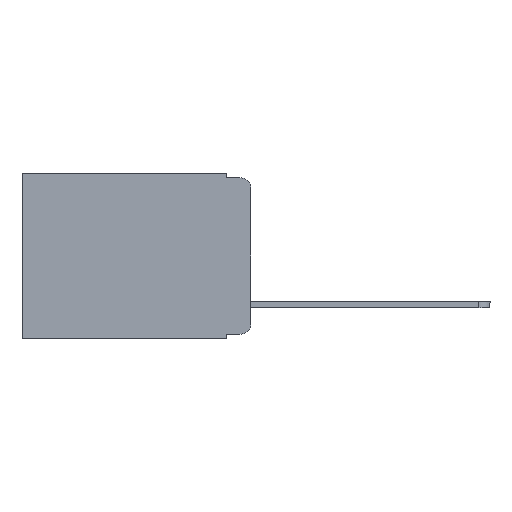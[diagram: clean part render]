
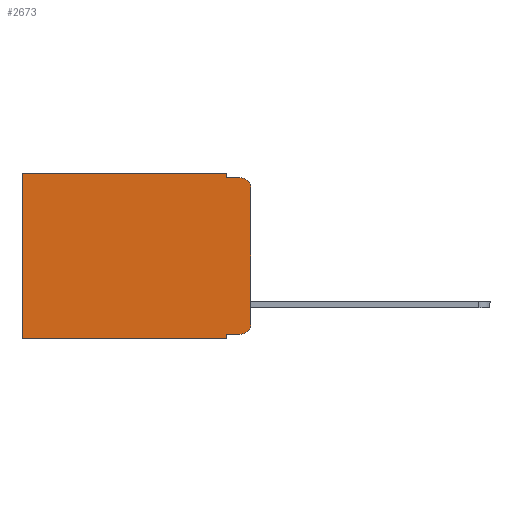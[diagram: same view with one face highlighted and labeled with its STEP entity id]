
A CAD part, left-side view. The second image highlights one B-rep face of the part: STEP entity #2673.
In plain terms, the highlighted planar face has unit normal (-1, 0, 0).
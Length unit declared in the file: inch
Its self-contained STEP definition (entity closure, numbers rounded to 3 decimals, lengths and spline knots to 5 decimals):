
#944 = VECTOR ( 'NONE', #15395, 39.37008 ) ;
#1008 = VERTEX_POINT ( 'NONE', #15096 ) ;
#1097 = DIRECTION ( 'NONE',  ( 0., 0., -1. ) ) ;
#1245 = VECTOR ( 'NONE', #19714, 39.37008 ) ;
#1649 = EDGE_CURVE ( 'NONE', #9801, #5990, #6736, .T. ) ;
#1655 = DIRECTION ( 'NONE',  ( 0., 0., -1. ) ) ;
#1959 = VERTEX_POINT ( 'NONE', #6568 ) ;
#2218 = EDGE_CURVE ( 'NONE', #9801, #3393, #4034, .T. ) ;
#2263 = CARTESIAN_POINT ( 'NONE',  ( 0.298, 0.02, -0.333 ) ) ;
#2331 = ORIENTED_EDGE ( 'NONE', *, *, #2218, .F. ) ;
#2642 = VECTOR ( 'NONE', #21369, 39.37008 ) ;
#2658 = EDGE_CURVE ( 'NONE', #5990, #1959, #10493, .T. ) ;
#2673 = ADVANCED_FACE ( 'NONE', ( #18002 ), #17777, .F. ) ;
#3393 = VERTEX_POINT ( 'NONE', #3511 ) ;
#3511 = CARTESIAN_POINT ( 'NONE',  ( 0.298, 0.051, -0.343 ) ) ;
#3837 = EDGE_LOOP ( 'NONE', ( #21745, #6970, #10984, #18626, #10590, #21558, #14095, #2331, #8886, #9224 ) ) ;
#4034 = LINE ( 'NONE', #4265, #10787 ) ;
#4265 = CARTESIAN_POINT ( 'NONE',  ( 0.298, 0.051, 0. ) ) ;
#5138 = CARTESIAN_POINT ( 'NONE',  ( 0.298, 0.051, -0.333 ) ) ;
#5890 = VECTOR ( 'NONE', #20852, 39.37008 ) ;
#5990 = VERTEX_POINT ( 'NONE', #2263 ) ;
#6135 = CARTESIAN_POINT ( 'NONE',  ( 0.298, 0.051, -0.01 ) ) ;
#6185 = DIRECTION ( 'NONE',  ( 0., 0., -1. ) ) ;
#6568 = CARTESIAN_POINT ( 'NONE',  ( 0.298, 0., -0.313 ) ) ;
#6736 = LINE ( 'NONE', #5138, #944 ) ;
#6970 = ORIENTED_EDGE ( 'NONE', *, *, #21407, .T. ) ;
#7196 = VERTEX_POINT ( 'NONE', #8000 ) ;
#7890 = CARTESIAN_POINT ( 'NONE',  ( 0.298, 0., 0. ) ) ;
#8000 = CARTESIAN_POINT ( 'NONE',  ( 0.298, 0.02, -0.01 ) ) ;
#8391 = CARTESIAN_POINT ( 'NONE',  ( 0.298, 0.051, 0. ) ) ;
#8419 = CARTESIAN_POINT ( 'NONE',  ( 0.298, 0.473, -0.343 ) ) ;
#8500 = CARTESIAN_POINT ( 'NONE',  ( 0.298, 0.473, 0. ) ) ;
#8886 = ORIENTED_EDGE ( 'NONE', *, *, #1649, .T. ) ;
#8892 = EDGE_CURVE ( 'NONE', #18422, #7196, #21714, .T. ) ;
#8947 = LINE ( 'NONE', #12167, #9162 ) ;
#9162 = VECTOR ( 'NONE', #22509, 39.37008 ) ;
#9224 = ORIENTED_EDGE ( 'NONE', *, *, #2658, .T. ) ;
#9284 = AXIS2_PLACEMENT_3D ( 'NONE', #12581, #17235, #1655 ) ;
#9745 = LINE ( 'NONE', #16690, #11934 ) ;
#9801 = VERTEX_POINT ( 'NONE', #18343 ) ;
#10105 = VECTOR ( 'NONE', #22389, 39.37008 ) ;
#10493 = CIRCLE ( 'NONE', #19944, 0.02 ) ;
#10590 = ORIENTED_EDGE ( 'NONE', *, *, #17525, .T. ) ;
#10622 = EDGE_CURVE ( 'NONE', #20757, #18422, #9745, .T. ) ;
#10787 = VECTOR ( 'NONE', #12949, 39.37008 ) ;
#10984 = ORIENTED_EDGE ( 'NONE', *, *, #8892, .F. ) ;
#11254 = VERTEX_POINT ( 'NONE', #17663 ) ;
#11306 = LINE ( 'NONE', #12683, #1245 ) ;
#11934 = VECTOR ( 'NONE', #1097, 39.37008 ) ;
#12167 = CARTESIAN_POINT ( 'NONE',  ( 0.298, 0., 0. ) ) ;
#12581 = CARTESIAN_POINT ( 'NONE',  ( 0.298, 0.02, -0.03 ) ) ;
#12683 = CARTESIAN_POINT ( 'NONE',  ( 0.298, 0., -0.343 ) ) ;
#12922 = DIRECTION ( 'NONE',  ( 1., 0., 0. ) ) ;
#12949 = DIRECTION ( 'NONE',  ( 0., 0., -1. ) ) ;
#13025 = EDGE_CURVE ( 'NONE', #11254, #22288, #19289, .T. ) ;
#13443 = AXIS2_PLACEMENT_3D ( 'NONE', #7890, #12922, #6185 ) ;
#14095 = ORIENTED_EDGE ( 'NONE', *, *, #20208, .F. ) ;
#14748 = DIRECTION ( 'NONE',  ( -1., 0., 0. ) ) ;
#14857 = CARTESIAN_POINT ( 'NONE',  ( 0.298, 0.02, -0.313 ) ) ;
#15096 = CARTESIAN_POINT ( 'NONE',  ( 0.298, 0., -0.03 ) ) ;
#15395 = DIRECTION ( 'NONE',  ( 0., -1., 0. ) ) ;
#16690 = CARTESIAN_POINT ( 'NONE',  ( 0.298, 0.051, 0. ) ) ;
#16909 = CIRCLE ( 'NONE', #9284, 0.02 ) ;
#17235 = DIRECTION ( 'NONE',  ( -1., 0., 0. ) ) ;
#17525 = EDGE_CURVE ( 'NONE', #20757, #11254, #22346, .T. ) ;
#17663 = CARTESIAN_POINT ( 'NONE',  ( 0.298, 0.473, 0. ) ) ;
#17777 = PLANE ( 'NONE',  #13443 ) ;
#18002 = FACE_OUTER_BOUND ( 'NONE', #3837, .T. ) ;
#18343 = CARTESIAN_POINT ( 'NONE',  ( 0.298, 0.051, -0.333 ) ) ;
#18422 = VERTEX_POINT ( 'NONE', #18857 ) ;
#18548 = EDGE_CURVE ( 'NONE', #1008, #1959, #8947, .T. ) ;
#18626 = ORIENTED_EDGE ( 'NONE', *, *, #10622, .F. ) ;
#18800 = CARTESIAN_POINT ( 'NONE',  ( 0.298, 0., 0. ) ) ;
#18857 = CARTESIAN_POINT ( 'NONE',  ( 0.298, 0.051, -0.01 ) ) ;
#19289 = LINE ( 'NONE', #8500, #10105 ) ;
#19714 = DIRECTION ( 'NONE',  ( 0., 1., 0. ) ) ;
#19944 = AXIS2_PLACEMENT_3D ( 'NONE', #14857, #14748, #21765 ) ;
#20208 = EDGE_CURVE ( 'NONE', #3393, #22288, #11306, .T. ) ;
#20757 = VERTEX_POINT ( 'NONE', #8391 ) ;
#20852 = DIRECTION ( 'NONE',  ( 0., 1., 0. ) ) ;
#21369 = DIRECTION ( 'NONE',  ( 0., -1., 0. ) ) ;
#21407 = EDGE_CURVE ( 'NONE', #1008, #7196, #16909, .T. ) ;
#21558 = ORIENTED_EDGE ( 'NONE', *, *, #13025, .T. ) ;
#21714 = LINE ( 'NONE', #6135, #2642 ) ;
#21745 = ORIENTED_EDGE ( 'NONE', *, *, #18548, .F. ) ;
#21765 = DIRECTION ( 'NONE',  ( 0., 0., -1. ) ) ;
#22288 = VERTEX_POINT ( 'NONE', #8419 ) ;
#22346 = LINE ( 'NONE', #18800, #5890 ) ;
#22389 = DIRECTION ( 'NONE',  ( 0., 0., -1. ) ) ;
#22509 = DIRECTION ( 'NONE',  ( 0., 0., -1. ) ) ;
